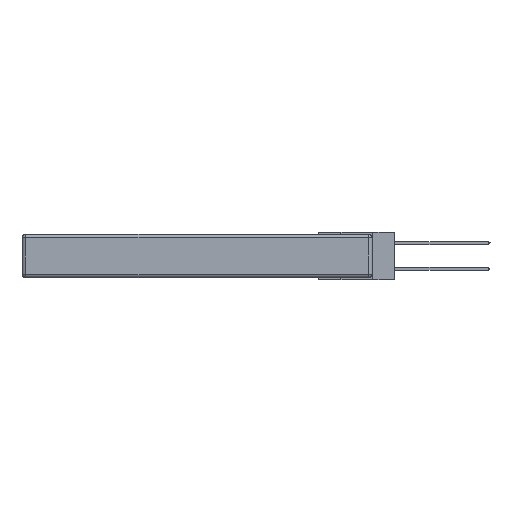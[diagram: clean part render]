
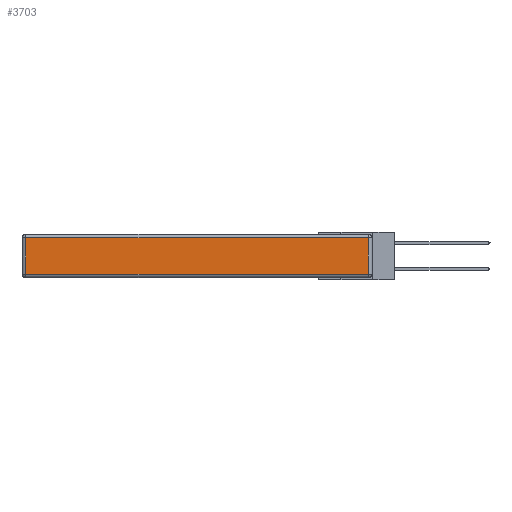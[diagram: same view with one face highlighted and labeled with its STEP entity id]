
A CAD part, left-side view. The second image highlights one B-rep face of the part: STEP entity #3703.
In plain terms, the highlighted planar face has unit normal (-1, 0, 0).
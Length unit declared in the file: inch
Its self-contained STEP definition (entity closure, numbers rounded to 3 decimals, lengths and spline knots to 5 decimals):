
#311 = VERTEX_POINT ( 'NONE', #15544 ) ;
#1677 = CARTESIAN_POINT ( 'NONE',  ( 0., 0.03, -0.343 ) ) ;
#3703 = ADVANCED_FACE ( 'NONE', ( #22247 ), #17513, .T. ) ;
#5289 = DIRECTION ( 'NONE',  ( -1., 0., 0. ) ) ;
#6391 = EDGE_CURVE ( 'NONE', #27966, #12170, #29314, .T. ) ;
#7139 = CARTESIAN_POINT ( 'NONE',  ( 0., 0.03, -0.313 ) ) ;
#9992 = ORIENTED_EDGE ( 'NONE', *, *, #19321, .T. ) ;
#10033 = CARTESIAN_POINT ( 'NONE',  ( 0., 0., -0.343 ) ) ;
#11289 = ORIENTED_EDGE ( 'NONE', *, *, #29487, .T. ) ;
#12170 = VERTEX_POINT ( 'NONE', #15961 ) ;
#12178 = VECTOR ( 'NONE', #22030, 39.37008 ) ;
#12529 = LINE ( 'NONE', #29019, #15975 ) ;
#12839 = ORIENTED_EDGE ( 'NONE', *, *, #25323, .T. ) ;
#13812 = EDGE_LOOP ( 'NONE', ( #12839, #11289, #9992, #15057 ) ) ;
#13910 = DIRECTION ( 'NONE',  ( 0., 0., 1. ) ) ;
#15057 = ORIENTED_EDGE ( 'NONE', *, *, #6391, .T. ) ;
#15544 = CARTESIAN_POINT ( 'NONE',  ( 0., 0.03, -0.03 ) ) ;
#15785 = VECTOR ( 'NONE', #21602, 39.37008 ) ;
#15961 = CARTESIAN_POINT ( 'NONE',  ( 0., 2.72, -0.313 ) ) ;
#15975 = VECTOR ( 'NONE', #21455, 39.37008 ) ;
#16667 = VECTOR ( 'NONE', #13910, 39.37008 ) ;
#16907 = LINE ( 'NONE', #31220, #15785 ) ;
#17407 = DIRECTION ( 'NONE',  ( 0., 0., 1. ) ) ;
#17513 = PLANE ( 'NONE',  #24321 ) ;
#17778 = LINE ( 'NONE', #1677, #16667 ) ;
#19321 = EDGE_CURVE ( 'NONE', #311, #27966, #16907, .T. ) ;
#21297 = VERTEX_POINT ( 'NONE', #7139 ) ;
#21455 = DIRECTION ( 'NONE',  ( 0., -1., 0. ) ) ;
#21602 = DIRECTION ( 'NONE',  ( 0., 1., 0. ) ) ;
#22030 = DIRECTION ( 'NONE',  ( 0., 0., -1. ) ) ;
#22247 = FACE_OUTER_BOUND ( 'NONE', #13812, .T. ) ;
#24321 = AXIS2_PLACEMENT_3D ( 'NONE', #10033, #5289, #17407 ) ;
#25323 = EDGE_CURVE ( 'NONE', #12170, #21297, #12529, .T. ) ;
#27966 = VERTEX_POINT ( 'NONE', #28087 ) ;
#28087 = CARTESIAN_POINT ( 'NONE',  ( 0., 2.72, -0.03 ) ) ;
#28766 = CARTESIAN_POINT ( 'NONE',  ( 0., 2.72, -0.343 ) ) ;
#29019 = CARTESIAN_POINT ( 'NONE',  ( 0., 0., -0.313 ) ) ;
#29314 = LINE ( 'NONE', #28766, #12178 ) ;
#29487 = EDGE_CURVE ( 'NONE', #21297, #311, #17778, .T. ) ;
#31220 = CARTESIAN_POINT ( 'NONE',  ( 0., 2.75, -0.03 ) ) ;
